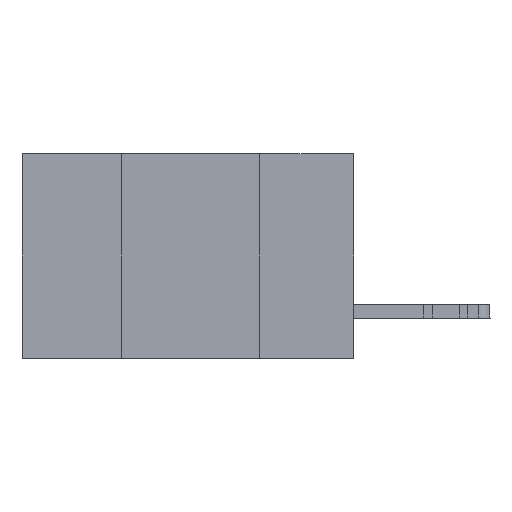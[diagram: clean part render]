
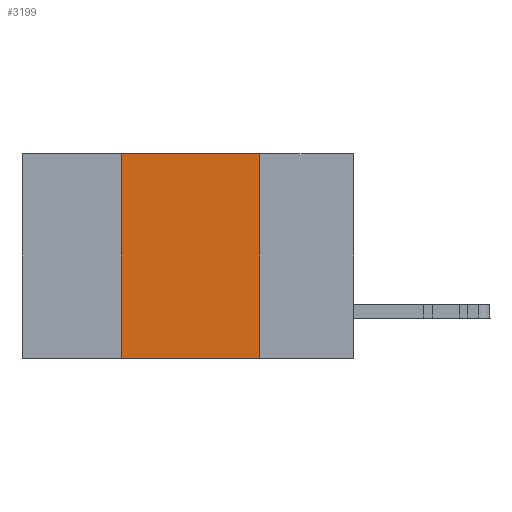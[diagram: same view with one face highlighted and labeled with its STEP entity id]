
A CAD part, left-side view. The second image highlights one B-rep face of the part: STEP entity #3199.
In plain terms, the highlighted planar face has unit normal (-1, 0, 0).
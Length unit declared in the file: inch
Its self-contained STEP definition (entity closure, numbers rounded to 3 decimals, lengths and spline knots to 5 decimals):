
#111 = VERTEX_POINT ( 'NONE', #36223 ) ;
#2263 = VECTOR ( 'NONE', #17266, 39.37008 ) ;
#3199 = ADVANCED_FACE ( 'NONE', ( #24784 ), #35973, .F. ) ;
#3820 = LINE ( 'NONE', #40918, #2263 ) ;
#3927 = CARTESIAN_POINT ( 'NONE',  ( 0., 0.42, -0.37 ) ) ;
#4930 = EDGE_CURVE ( 'NONE', #40863, #40047, #12075, .T. ) ;
#9594 = CARTESIAN_POINT ( 'NONE',  ( 0., 0.6, 0. ) ) ;
#11484 = VERTEX_POINT ( 'NONE', #12115 ) ;
#11683 = ORIENTED_EDGE ( 'NONE', *, *, #4930, .T. ) ;
#12075 = LINE ( 'NONE', #16900, #37678 ) ;
#12115 = CARTESIAN_POINT ( 'NONE',  ( 0., 0.42, 0. ) ) ;
#16597 = DIRECTION ( 'NONE',  ( 0., -1., 0. ) ) ;
#16900 = CARTESIAN_POINT ( 'NONE',  ( 0., 0.6, -0.37 ) ) ;
#17266 = DIRECTION ( 'NONE',  ( 0., 0., -1. ) ) ;
#18278 = EDGE_CURVE ( 'NONE', #40863, #11484, #30540, .T. ) ;
#20487 = ORIENTED_EDGE ( 'NONE', *, *, #18278, .F. ) ;
#24784 = FACE_OUTER_BOUND ( 'NONE', #27831, .T. ) ;
#25542 = EDGE_CURVE ( 'NONE', #111, #40047, #3820, .T. ) ;
#27690 = AXIS2_PLACEMENT_3D ( 'NONE', #9594, #39785, #35829 ) ;
#27831 = EDGE_LOOP ( 'NONE', ( #31408, #41796, #20487, #11683 ) ) ;
#29468 = CARTESIAN_POINT ( 'NONE',  ( 0., 0.17, -0.37 ) ) ;
#30327 = DIRECTION ( 'NONE',  ( 0., -1., 0. ) ) ;
#30540 = LINE ( 'NONE', #42372, #35743 ) ;
#31408 = ORIENTED_EDGE ( 'NONE', *, *, #25542, .F. ) ;
#34216 = LINE ( 'NONE', #36729, #42057 ) ;
#35538 = EDGE_CURVE ( 'NONE', #11484, #111, #34216, .T. ) ;
#35743 = VECTOR ( 'NONE', #38863, 39.37008 ) ;
#35829 = DIRECTION ( 'NONE',  ( 0., 0., -1. ) ) ;
#35973 = PLANE ( 'NONE',  #27690 ) ;
#36223 = CARTESIAN_POINT ( 'NONE',  ( 0., 0.17, 0. ) ) ;
#36729 = CARTESIAN_POINT ( 'NONE',  ( 0., 0.6, 0. ) ) ;
#37678 = VECTOR ( 'NONE', #30327, 39.37008 ) ;
#38863 = DIRECTION ( 'NONE',  ( 0., 0., 1. ) ) ;
#39785 = DIRECTION ( 'NONE',  ( 1., 0., 0. ) ) ;
#40047 = VERTEX_POINT ( 'NONE', #29468 ) ;
#40863 = VERTEX_POINT ( 'NONE', #3927 ) ;
#40918 = CARTESIAN_POINT ( 'NONE',  ( 0., 0.17, 0. ) ) ;
#41796 = ORIENTED_EDGE ( 'NONE', *, *, #35538, .F. ) ;
#42057 = VECTOR ( 'NONE', #16597, 39.37008 ) ;
#42372 = CARTESIAN_POINT ( 'NONE',  ( 0., 0.42, 0. ) ) ;
